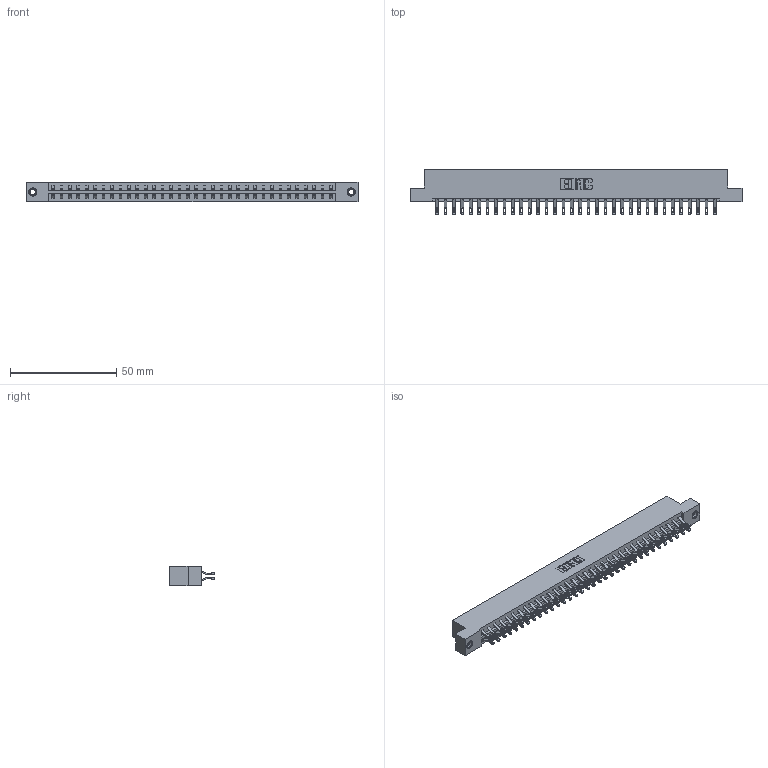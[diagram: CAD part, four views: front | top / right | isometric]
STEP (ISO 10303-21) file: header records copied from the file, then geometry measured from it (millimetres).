
FILE_DESCRIPTION (( 'STEP AP203' ), '1' );
FILE_NAME ('833-068-555-207.STEP', '2020-06-05T11:05:07', ( '' ), ( '' ), 'SwSTEP 2.0', 'SolidWorks 2020', '' );
FILE_SCHEMA (( 'CONFIG_CONTROL_DESIGN' ));
Length unit declared in the file: inch
Products named in the file (4): 345-292-001_555 Tail; 833-068-555-207; 833 Part_Flush - .156 Dia - TI; 345-250-001_345-250-005-103
Assembly tree (71 placements, depth 2):
  833-068-555-207
    833 Part_Flush - .156 Dia - TI
    345-292-001_555 Tail  x68
    345-250-001_345-250-005-103  x2
Bounding box: 156.26 x 21.47 x 9.4 mm (x, y, z)
Volume: 16062.2 mm3; surface area: 19675.4 mm2
Topology: 71 solids, 71 shells, 4118 faces, 12891 edges, 8586 vertices
Faces by surface type: plane 2414, cylinder 1688, cone 12, torus 4
Entity records: 24420 total; most frequent: CARTESIAN_POINT 4075, ORIENTED_EDGE 3974, DIRECTION 3497, EDGE_CURVE 1987, VECTOR 1819, LINE 1819, VERTEX_POINT 1320, AXIS2_PLACEMENT_3D 839
